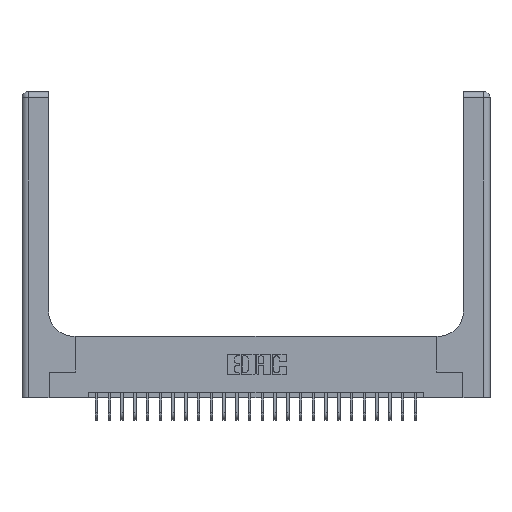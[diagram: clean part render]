
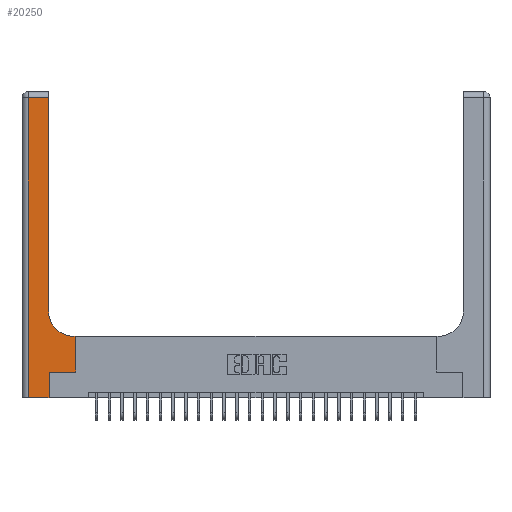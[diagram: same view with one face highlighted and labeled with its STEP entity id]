
A CAD part, top view. The second image highlights one B-rep face of the part: STEP entity #20250.
In plain terms, the highlighted planar face has unit normal (0, 0, 1).
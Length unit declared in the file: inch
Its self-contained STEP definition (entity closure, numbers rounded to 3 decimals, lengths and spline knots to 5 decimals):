
#170 = EDGE_CURVE ( 'NONE', #26405, #11214, #8468, .T. ) ;
#1043 = DIRECTION ( 'NONE',  ( 1., 0., 0. ) ) ;
#1060 = LINE ( 'NONE', #25652, #19696 ) ;
#1294 = CARTESIAN_POINT ( 'NONE',  ( 0.528, 0.25, 0.37 ) ) ;
#1402 = EDGE_CURVE ( 'NONE', #14864, #17443, #2057, .T. ) ;
#1648 = DIRECTION ( 'NONE',  ( 0., 1., 0. ) ) ;
#1788 = DIRECTION ( 'NONE',  ( -1., 0., 0. ) ) ;
#1914 = CARTESIAN_POINT ( 'NONE',  ( 0.265, 0., 0.37 ) ) ;
#2057 = LINE ( 'NONE', #26134, #6559 ) ;
#2254 = VERTEX_POINT ( 'NONE', #6649 ) ;
#2423 = CARTESIAN_POINT ( 'NONE',  ( 0.51, 0.6, 0.37 ) ) ;
#3111 = CIRCLE ( 'NONE', #26295, 0.25 ) ;
#3537 = ORIENTED_EDGE ( 'NONE', *, *, #1402, .T. ) ;
#3586 = DIRECTION ( 'NONE',  ( 0., -1., 0. ) ) ;
#4119 = LINE ( 'NONE', #20652, #4900 ) ;
#4900 = VECTOR ( 'NONE', #14347, 39.37008 ) ;
#5163 = EDGE_CURVE ( 'NONE', #6251, #18797, #17926, .T. ) ;
#5192 = DIRECTION ( 'NONE',  ( 0., 0., -1. ) ) ;
#6016 = ORIENTED_EDGE ( 'NONE', *, *, #18140, .T. ) ;
#6246 = EDGE_CURVE ( 'NONE', #18797, #13753, #6812, .T. ) ;
#6251 = VERTEX_POINT ( 'NONE', #17166 ) ;
#6559 = VECTOR ( 'NONE', #1788, 39.37008 ) ;
#6649 = CARTESIAN_POINT ( 'NONE',  ( 0.06, 0., 0.37 ) ) ;
#6812 = LINE ( 'NONE', #11243, #14652 ) ;
#6838 = CARTESIAN_POINT ( 'NONE',  ( 0.26, 0.85, 0.37 ) ) ;
#6861 = CARTESIAN_POINT ( 'NONE',  ( 0., 3., 0.37 ) ) ;
#7268 = EDGE_CURVE ( 'NONE', #17443, #26405, #3111, .T. ) ;
#8024 = CARTESIAN_POINT ( 'NONE',  ( 0.06, 2.94, 0.37 ) ) ;
#8468 = LINE ( 'NONE', #18691, #14323 ) ;
#10617 = DIRECTION ( 'NONE',  ( 0., 1., 0. ) ) ;
#10724 = LINE ( 'NONE', #25238, #25973 ) ;
#11214 = VERTEX_POINT ( 'NONE', #17656 ) ;
#11243 = CARTESIAN_POINT ( 'NONE',  ( 0.265, 0.25, 0.37 ) ) ;
#11399 = CARTESIAN_POINT ( 'NONE',  ( 0.528, 0.6, 0.37 ) ) ;
#12271 = EDGE_CURVE ( 'NONE', #11214, #16434, #10724, .T. ) ;
#12559 = ORIENTED_EDGE ( 'NONE', *, *, #24489, .T. ) ;
#13180 = ORIENTED_EDGE ( 'NONE', *, *, #12271, .T. ) ;
#13753 = VERTEX_POINT ( 'NONE', #1294 ) ;
#14323 = VECTOR ( 'NONE', #10617, 39.37008 ) ;
#14347 = DIRECTION ( 'NONE',  ( 1., 0., 0. ) ) ;
#14652 = VECTOR ( 'NONE', #15027, 39.37008 ) ;
#14864 = VERTEX_POINT ( 'NONE', #11399 ) ;
#14951 = PLANE ( 'NONE',  #16365 ) ;
#15026 = EDGE_LOOP ( 'NONE', ( #16673, #13180, #6016, #19920, #15968, #18700, #12559, #3537, #16018 ) ) ;
#15027 = DIRECTION ( 'NONE',  ( 1., 0., 0. ) ) ;
#15968 = ORIENTED_EDGE ( 'NONE', *, *, #5163, .T. ) ;
#16018 = ORIENTED_EDGE ( 'NONE', *, *, #7268, .T. ) ;
#16365 = AXIS2_PLACEMENT_3D ( 'NONE', #6861, #21868, #17858 ) ;
#16434 = VERTEX_POINT ( 'NONE', #8024 ) ;
#16673 = ORIENTED_EDGE ( 'NONE', *, *, #170, .T. ) ;
#16991 = LINE ( 'NONE', #19277, #19533 ) ;
#17166 = CARTESIAN_POINT ( 'NONE',  ( 0.265, 0., 0.37 ) ) ;
#17249 = DIRECTION ( 'NONE',  ( 0., 1., 0. ) ) ;
#17443 = VERTEX_POINT ( 'NONE', #2423 ) ;
#17656 = CARTESIAN_POINT ( 'NONE',  ( 0.26, 2.94, 0.37 ) ) ;
#17858 = DIRECTION ( 'NONE',  ( -1., 0., 0. ) ) ;
#17926 = LINE ( 'NONE', #1914, #19780 ) ;
#17997 = FACE_OUTER_BOUND ( 'NONE', #15026, .T. ) ;
#18140 = EDGE_CURVE ( 'NONE', #16434, #2254, #1060, .T. ) ;
#18691 = CARTESIAN_POINT ( 'NONE',  ( 0.26, 3., 0.37 ) ) ;
#18700 = ORIENTED_EDGE ( 'NONE', *, *, #6246, .T. ) ;
#18797 = VERTEX_POINT ( 'NONE', #20152 ) ;
#19277 = CARTESIAN_POINT ( 'NONE',  ( 0.528, 0.25, 0.37 ) ) ;
#19533 = VECTOR ( 'NONE', #17249, 39.37008 ) ;
#19696 = VECTOR ( 'NONE', #3586, 39.37008 ) ;
#19780 = VECTOR ( 'NONE', #1648, 39.37008 ) ;
#19920 = ORIENTED_EDGE ( 'NONE', *, *, #25480, .T. ) ;
#20152 = CARTESIAN_POINT ( 'NONE',  ( 0.265, 0.25, 0.37 ) ) ;
#20250 = ADVANCED_FACE ( 'NONE', ( #17997 ), #14951, .F. ) ;
#20652 = CARTESIAN_POINT ( 'NONE',  ( 0., 0., 0.37 ) ) ;
#21063 = DIRECTION ( 'NONE',  ( -1., 0., 0. ) ) ;
#21868 = DIRECTION ( 'NONE',  ( 0., 0., -1. ) ) ;
#23605 = CARTESIAN_POINT ( 'NONE',  ( 0.51, 0.85, 0.37 ) ) ;
#24489 = EDGE_CURVE ( 'NONE', #13753, #14864, #16991, .T. ) ;
#25238 = CARTESIAN_POINT ( 'NONE',  ( 0., 2.94, 0.37 ) ) ;
#25480 = EDGE_CURVE ( 'NONE', #2254, #6251, #4119, .T. ) ;
#25652 = CARTESIAN_POINT ( 'NONE',  ( 0.06, 3., 0.37 ) ) ;
#25973 = VECTOR ( 'NONE', #21063, 39.37008 ) ;
#26134 = CARTESIAN_POINT ( 'NONE',  ( 0.26, 0.6, 0.37 ) ) ;
#26295 = AXIS2_PLACEMENT_3D ( 'NONE', #23605, #5192, #1043 ) ;
#26405 = VERTEX_POINT ( 'NONE', #6838 ) ;
